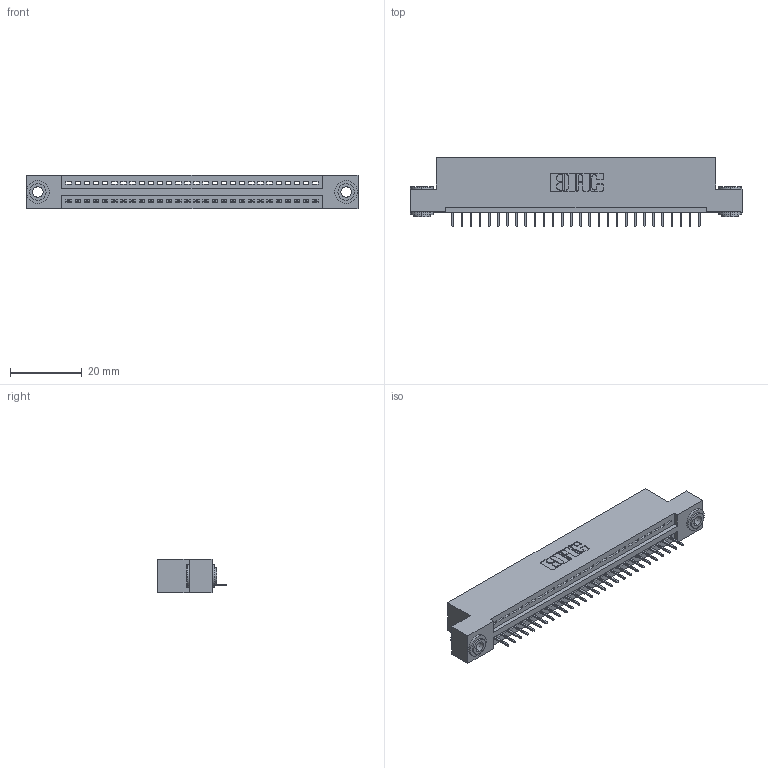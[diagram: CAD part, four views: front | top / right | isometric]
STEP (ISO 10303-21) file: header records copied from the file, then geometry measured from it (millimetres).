
FILE_DESCRIPTION (( 'STEP AP203' ), '1' );
FILE_NAME ('395-028-524-103.STEP', '2018-11-10T09:44:48', ( '' ), ( '' ), 'SwSTEP 2.0', 'SolidWorks 2016', '' );
FILE_SCHEMA (( 'CONFIG_CONTROL_DESIGN' ));
Length unit declared in the file: inch
Products named in the file (4): 345-250-002_345-250-002-102; 345-292-001_345-293-124; 395-028-524-103; 345 Part_Flush Mounting Lugs - 0.156 Dia-TH
Assembly tree (31 placements, depth 2):
  395-028-524-103
    345 Part_Flush Mounting Lugs - 0.156 Dia-TH
    345-292-001_345-293-124  x28
    345-250-002_345-250-002-102  x2
Bounding box: 92.33 x 19.35 x 9.4 mm (x, y, z)
Volume: 8563.6 mm3; surface area: 11050.8 mm2
Topology: 31 solids, 31 shells, 1900 faces, 5457 edges, 3522 vertices
Faces by surface type: plane 1378, cylinder 514, cone 8
Entity records: 23682 total; most frequent: CARTESIAN_POINT 4079, ORIENTED_EDGE 4034, DIRECTION 3615, EDGE_CURVE 2017, LINE 1753, VECTOR 1753, VERTEX_POINT 1338, AXIS2_PLACEMENT_3D 931
